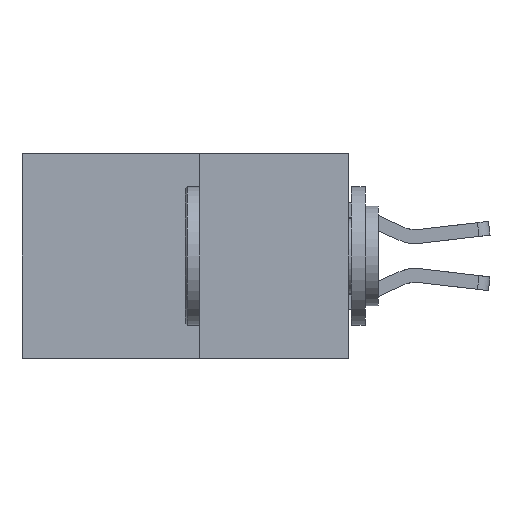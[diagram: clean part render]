
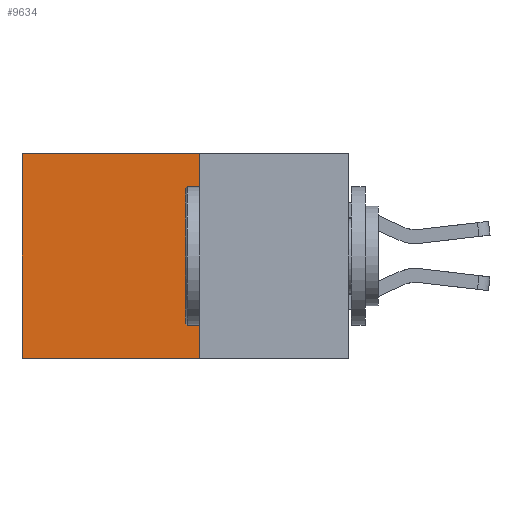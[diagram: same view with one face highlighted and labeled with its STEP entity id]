
A CAD part, left-side view. The second image highlights one B-rep face of the part: STEP entity #9634.
In plain terms, the highlighted planar face has unit normal (-1, 0, 0).
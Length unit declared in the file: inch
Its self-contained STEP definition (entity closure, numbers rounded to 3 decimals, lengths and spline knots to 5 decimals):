
#235 = VECTOR ( 'NONE', #9856, 39.37008 ) ;
#575 = AXIS2_PLACEMENT_3D ( 'NONE', #3201, #4033, #9518 ) ;
#673 = ORIENTED_EDGE ( 'NONE', *, *, #6353, .F. ) ;
#987 = VERTEX_POINT ( 'NONE', #6429 ) ;
#1351 = CARTESIAN_POINT ( 'NONE',  ( 0.277, 0.27, 0. ) ) ;
#2205 = VERTEX_POINT ( 'NONE', #4197 ) ;
#2691 = CARTESIAN_POINT ( 'NONE',  ( 0.277, 0.27, 0. ) ) ;
#2813 = DIRECTION ( 'NONE',  ( 0., 1., 0. ) ) ;
#3111 = FACE_OUTER_BOUND ( 'NONE', #7096, .T. ) ;
#3140 = VECTOR ( 'NONE', #2813, 39.37008 ) ;
#3201 = CARTESIAN_POINT ( 'NONE',  ( 0.277, 0.27, -0.37 ) ) ;
#3897 = DIRECTION ( 'NONE',  ( 0., 0., -1. ) ) ;
#4022 = CARTESIAN_POINT ( 'NONE',  ( 0.277, 0.27, -0.37 ) ) ;
#4033 = DIRECTION ( 'NONE',  ( 1., 0., 0. ) ) ;
#4085 = EDGE_CURVE ( 'NONE', #6493, #2205, #10383, .T. ) ;
#4197 = CARTESIAN_POINT ( 'NONE',  ( 0.277, 0.27, -0.37 ) ) ;
#4204 = EDGE_CURVE ( 'NONE', #6493, #987, #5273, .T. ) ;
#4558 = EDGE_CURVE ( 'NONE', #987, #8145, #5396, .T. ) ;
#5159 = ORIENTED_EDGE ( 'NONE', *, *, #4085, .F. ) ;
#5273 = LINE ( 'NONE', #2691, #3140 ) ;
#5396 = LINE ( 'NONE', #9909, #235 ) ;
#5733 = VECTOR ( 'NONE', #8646, 39.37008 ) ;
#6275 = CARTESIAN_POINT ( 'NONE',  ( 0.277, 0.59, -0.37 ) ) ;
#6353 = EDGE_CURVE ( 'NONE', #2205, #8145, #7367, .T. ) ;
#6429 = CARTESIAN_POINT ( 'NONE',  ( 0.277, 0.59, 0. ) ) ;
#6493 = VERTEX_POINT ( 'NONE', #1351 ) ;
#7096 = EDGE_LOOP ( 'NONE', ( #7297, #673, #5159, #7519 ) ) ;
#7297 = ORIENTED_EDGE ( 'NONE', *, *, #4558, .T. ) ;
#7367 = LINE ( 'NONE', #8663, #5733 ) ;
#7519 = ORIENTED_EDGE ( 'NONE', *, *, #4204, .T. ) ;
#7984 = PLANE ( 'NONE',  #575 ) ;
#8145 = VERTEX_POINT ( 'NONE', #6275 ) ;
#8360 = VECTOR ( 'NONE', #3897, 39.37008 ) ;
#8646 = DIRECTION ( 'NONE',  ( 0., 1., 0. ) ) ;
#8663 = CARTESIAN_POINT ( 'NONE',  ( 0.277, 0.27, -0.37 ) ) ;
#9518 = DIRECTION ( 'NONE',  ( 0., 0., -1. ) ) ;
#9634 = ADVANCED_FACE ( 'NONE', ( #3111 ), #7984, .F. ) ;
#9856 = DIRECTION ( 'NONE',  ( 0., 0., -1. ) ) ;
#9909 = CARTESIAN_POINT ( 'NONE',  ( 0.277, 0.59, -0.37 ) ) ;
#10383 = LINE ( 'NONE', #4022, #8360 ) ;
